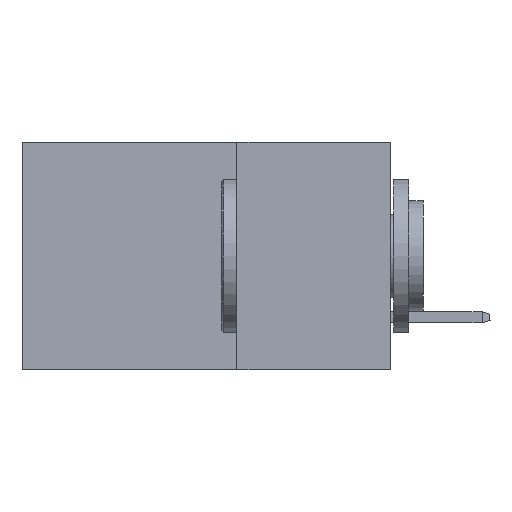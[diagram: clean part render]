
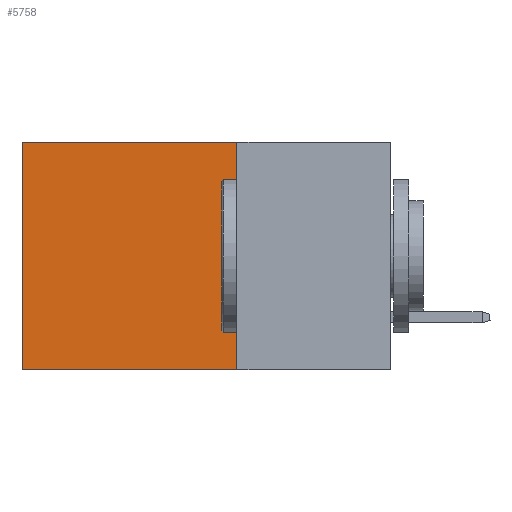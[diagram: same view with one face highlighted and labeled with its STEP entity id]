
A CAD part, left-side view. The second image highlights one B-rep face of the part: STEP entity #5758.
In plain terms, the highlighted planar face has unit normal (-1, 0, 0).
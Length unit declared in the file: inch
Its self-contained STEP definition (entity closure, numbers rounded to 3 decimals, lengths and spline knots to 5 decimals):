
#40 = DIRECTION ( 'NONE',  ( 0., 0., -1. ) ) ;
#679 = CARTESIAN_POINT ( 'NONE',  ( 0.2875, 0.25, 0. ) ) ;
#725 = DIRECTION ( 'NONE',  ( 0., 0., -1. ) ) ;
#1511 = ORIENTED_EDGE ( 'NONE', *, *, #3045, .T. ) ;
#1602 = PLANE ( 'NONE',  #2828 ) ;
#1999 = CARTESIAN_POINT ( 'NONE',  ( 0.2875, 0.6, 0. ) ) ;
#2128 = ORIENTED_EDGE ( 'NONE', *, *, #9102, .T. ) ;
#2177 = CARTESIAN_POINT ( 'NONE',  ( 0.2875, 0.25, 0. ) ) ;
#2828 = AXIS2_PLACEMENT_3D ( 'NONE', #3810, #6608, #725 ) ;
#2900 = LINE ( 'NONE', #1999, #12178 ) ;
#3045 = EDGE_CURVE ( 'NONE', #7394, #8872, #3800, .T. ) ;
#3800 = LINE ( 'NONE', #2177, #10776 ) ;
#3810 = CARTESIAN_POINT ( 'NONE',  ( 0.2875, 0.25, 0. ) ) ;
#4077 = VECTOR ( 'NONE', #8354, 39.37008 ) ;
#4229 = CARTESIAN_POINT ( 'NONE',  ( 0.2875, 0.6, 0. ) ) ;
#4349 = CARTESIAN_POINT ( 'NONE',  ( 0.2875, 0.25, 0. ) ) ;
#4765 = EDGE_CURVE ( 'NONE', #7394, #10607, #10257, .T. ) ;
#4963 = EDGE_CURVE ( 'NONE', #10607, #10909, #10403, .T. ) ;
#5363 = CARTESIAN_POINT ( 'NONE',  ( 0.2875, 0.6, -0.37 ) ) ;
#5697 = FACE_OUTER_BOUND ( 'NONE', #7133, .T. ) ;
#5758 = ADVANCED_FACE ( 'NONE', ( #5697 ), #1602, .F. ) ;
#6545 = ORIENTED_EDGE ( 'NONE', *, *, #4963, .F. ) ;
#6608 = DIRECTION ( 'NONE',  ( 1., 0., 0. ) ) ;
#6634 = DIRECTION ( 'NONE',  ( 0., 1., 0. ) ) ;
#6675 = CARTESIAN_POINT ( 'NONE',  ( 0.2875, 0.25, -0.37 ) ) ;
#7025 = ORIENTED_EDGE ( 'NONE', *, *, #4765, .F. ) ;
#7133 = EDGE_LOOP ( 'NONE', ( #2128, #6545, #7025, #1511 ) ) ;
#7394 = VERTEX_POINT ( 'NONE', #4349 ) ;
#8354 = DIRECTION ( 'NONE',  ( 0., 0., -1. ) ) ;
#8872 = VERTEX_POINT ( 'NONE', #4229 ) ;
#9102 = EDGE_CURVE ( 'NONE', #8872, #10909, #2900, .T. ) ;
#9155 = VECTOR ( 'NONE', #6634, 39.37008 ) ;
#9211 = DIRECTION ( 'NONE',  ( 0., 1., 0. ) ) ;
#10257 = LINE ( 'NONE', #679, #4077 ) ;
#10403 = LINE ( 'NONE', #11478, #9155 ) ;
#10607 = VERTEX_POINT ( 'NONE', #6675 ) ;
#10776 = VECTOR ( 'NONE', #9211, 39.37008 ) ;
#10909 = VERTEX_POINT ( 'NONE', #5363 ) ;
#11478 = CARTESIAN_POINT ( 'NONE',  ( 0.2875, 0.25, -0.37 ) ) ;
#12178 = VECTOR ( 'NONE', #40, 39.37008 ) ;
